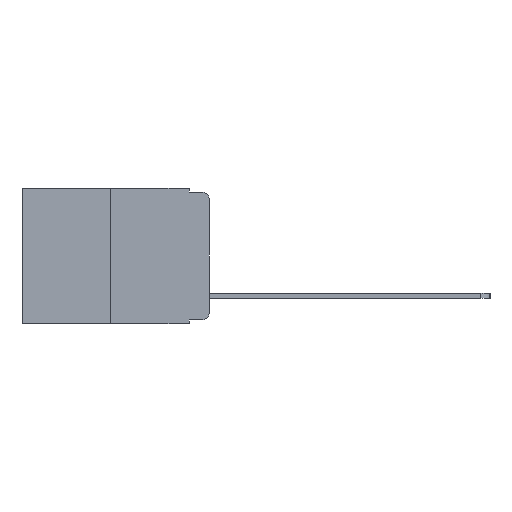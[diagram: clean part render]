
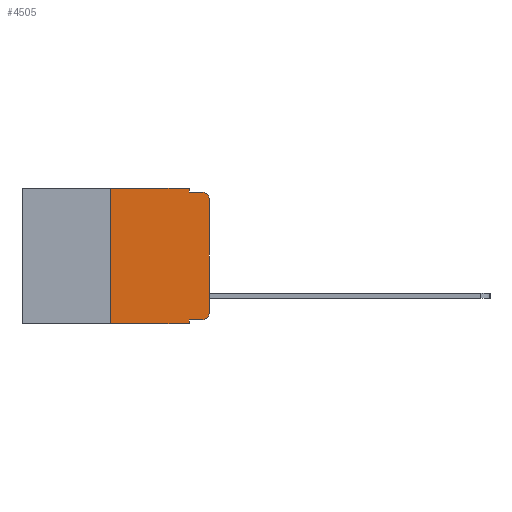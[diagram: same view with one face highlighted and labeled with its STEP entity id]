
A CAD part, left-side view. The second image highlights one B-rep face of the part: STEP entity #4505.
In plain terms, the highlighted planar face has unit normal (-1, 0, 0).
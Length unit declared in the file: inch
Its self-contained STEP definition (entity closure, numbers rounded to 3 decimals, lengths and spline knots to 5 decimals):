
#16 = EDGE_CURVE ( 'NONE', #2406, #8266, #8971, .T. ) ;
#35 = VERTEX_POINT ( 'NONE', #897 ) ;
#114 = ORIENTED_EDGE ( 'NONE', *, *, #5518, .F. ) ;
#208 = AXIS2_PLACEMENT_3D ( 'NONE', #2878, #8961, #3719 ) ;
#295 = CARTESIAN_POINT ( 'NONE',  ( 0., 0.051, 0. ) ) ;
#467 = ORIENTED_EDGE ( 'NONE', *, *, #7048, .F. ) ;
#675 = EDGE_CURVE ( 'NONE', #3174, #8266, #1093, .T. ) ;
#722 = VECTOR ( 'NONE', #9252, 39.37008 ) ;
#881 = LINE ( 'NONE', #295, #9978 ) ;
#897 = CARTESIAN_POINT ( 'NONE',  ( 0., 0.25, 0. ) ) ;
#975 = EDGE_CURVE ( 'NONE', #2092, #35, #4726, .T. ) ;
#1050 = LINE ( 'NONE', #3229, #722 ) ;
#1093 = LINE ( 'NONE', #2031, #4134 ) ;
#1581 = CARTESIAN_POINT ( 'NONE',  ( 0., 0.051, -0.333 ) ) ;
#2031 = CARTESIAN_POINT ( 'NONE',  ( 0., 0.051, -0.01 ) ) ;
#2092 = VERTEX_POINT ( 'NONE', #10854 ) ;
#2406 = VERTEX_POINT ( 'NONE', #10140 ) ;
#2514 = DIRECTION ( 'NONE',  ( 0., -1., 0. ) ) ;
#2523 = VERTEX_POINT ( 'NONE', #6070 ) ;
#2529 = CARTESIAN_POINT ( 'NONE',  ( 0., 0.051, -0.01 ) ) ;
#2704 = VECTOR ( 'NONE', #10367, 39.37008 ) ;
#2850 = ORIENTED_EDGE ( 'NONE', *, *, #3019, .F. ) ;
#2878 = CARTESIAN_POINT ( 'NONE',  ( 0., 0.02, -0.03 ) ) ;
#2907 = LINE ( 'NONE', #9374, #11278 ) ;
#2908 = DIRECTION ( 'NONE',  ( 0., -1., 0. ) ) ;
#3019 = EDGE_CURVE ( 'NONE', #9167, #3174, #881, .T. ) ;
#3174 = VERTEX_POINT ( 'NONE', #2529 ) ;
#3229 = CARTESIAN_POINT ( 'NONE',  ( 0., 0., 0. ) ) ;
#3245 = AXIS2_PLACEMENT_3D ( 'NONE', #5393, #3585, #8828 ) ;
#3280 = DIRECTION ( 'NONE',  ( -1., 0., 0. ) ) ;
#3315 = CARTESIAN_POINT ( 'NONE',  ( 0., 0.02, -0.313 ) ) ;
#3332 = VERTEX_POINT ( 'NONE', #1581 ) ;
#3585 = DIRECTION ( 'NONE',  ( 1., 0., 0. ) ) ;
#3594 = AXIS2_PLACEMENT_3D ( 'NONE', #3315, #3280, #9082 ) ;
#3719 = DIRECTION ( 'NONE',  ( 0., 0., -1. ) ) ;
#3962 = EDGE_CURVE ( 'NONE', #3332, #2523, #2907, .T. ) ;
#4134 = VECTOR ( 'NONE', #10295, 39.37008 ) ;
#4366 = FACE_OUTER_BOUND ( 'NONE', #8777, .T. ) ;
#4473 = CARTESIAN_POINT ( 'NONE',  ( 0., 0.051, 0. ) ) ;
#4491 = VECTOR ( 'NONE', #2514, 39.37008 ) ;
#4505 = ADVANCED_FACE ( 'NONE', ( #4366 ), #11149, .F. ) ;
#4626 = DIRECTION ( 'NONE',  ( 0., 0., 1. ) ) ;
#4726 = LINE ( 'NONE', #6317, #6840 ) ;
#4742 = LINE ( 'NONE', #9960, #11116 ) ;
#4773 = LINE ( 'NONE', #8956, #4491 ) ;
#4968 = EDGE_CURVE ( 'NONE', #2523, #9994, #10797, .T. ) ;
#5227 = CARTESIAN_POINT ( 'NONE',  ( 0., 0.02, -0.01 ) ) ;
#5393 = CARTESIAN_POINT ( 'NONE',  ( 0., 0.473, 0. ) ) ;
#5518 = EDGE_CURVE ( 'NONE', #35, #9167, #4773, .T. ) ;
#6070 = CARTESIAN_POINT ( 'NONE',  ( 0., 0.02, -0.333 ) ) ;
#6317 = CARTESIAN_POINT ( 'NONE',  ( 0., 0.25, 0. ) ) ;
#6396 = CARTESIAN_POINT ( 'NONE',  ( 0., 0.051, 0. ) ) ;
#6840 = VECTOR ( 'NONE', #4626, 39.37008 ) ;
#7048 = EDGE_CURVE ( 'NONE', #3332, #8185, #9332, .T. ) ;
#7272 = ORIENTED_EDGE ( 'NONE', *, *, #675, .F. ) ;
#7359 = DIRECTION ( 'NONE',  ( 0., -1., 0. ) ) ;
#7493 = EDGE_CURVE ( 'NONE', #2092, #8185, #4742, .T. ) ;
#7540 = ORIENTED_EDGE ( 'NONE', *, *, #7493, .T. ) ;
#8185 = VERTEX_POINT ( 'NONE', #9365 ) ;
#8266 = VERTEX_POINT ( 'NONE', #5227 ) ;
#8311 = ORIENTED_EDGE ( 'NONE', *, *, #3962, .T. ) ;
#8777 = EDGE_LOOP ( 'NONE', ( #11228, #9442, #7272, #2850, #114, #9687, #7540, #467, #8311, #10399 ) ) ;
#8828 = DIRECTION ( 'NONE',  ( 0., 0., -1. ) ) ;
#8846 = CARTESIAN_POINT ( 'NONE',  ( 0., 0., -0.313 ) ) ;
#8956 = CARTESIAN_POINT ( 'NONE',  ( 0., 0.473, 0. ) ) ;
#8961 = DIRECTION ( 'NONE',  ( -1., 0., 0. ) ) ;
#8971 = CIRCLE ( 'NONE', #208, 0.02 ) ;
#9082 = DIRECTION ( 'NONE',  ( 0., 0., -1. ) ) ;
#9167 = VERTEX_POINT ( 'NONE', #6396 ) ;
#9252 = DIRECTION ( 'NONE',  ( 0., 0., 1. ) ) ;
#9332 = LINE ( 'NONE', #4473, #2704 ) ;
#9365 = CARTESIAN_POINT ( 'NONE',  ( 0., 0.051, -0.343 ) ) ;
#9374 = CARTESIAN_POINT ( 'NONE',  ( 0., 0.051, -0.333 ) ) ;
#9442 = ORIENTED_EDGE ( 'NONE', *, *, #16, .T. ) ;
#9687 = ORIENTED_EDGE ( 'NONE', *, *, #975, .F. ) ;
#9960 = CARTESIAN_POINT ( 'NONE',  ( 0., 0.473, -0.343 ) ) ;
#9978 = VECTOR ( 'NONE', #10283, 39.37008 ) ;
#9994 = VERTEX_POINT ( 'NONE', #8846 ) ;
#10140 = CARTESIAN_POINT ( 'NONE',  ( 0., 0., -0.03 ) ) ;
#10283 = DIRECTION ( 'NONE',  ( 0., 0., -1. ) ) ;
#10295 = DIRECTION ( 'NONE',  ( 0., -1., 0. ) ) ;
#10367 = DIRECTION ( 'NONE',  ( 0., 0., -1. ) ) ;
#10399 = ORIENTED_EDGE ( 'NONE', *, *, #4968, .T. ) ;
#10497 = EDGE_CURVE ( 'NONE', #9994, #2406, #1050, .T. ) ;
#10797 = CIRCLE ( 'NONE', #3594, 0.02 ) ;
#10854 = CARTESIAN_POINT ( 'NONE',  ( 0., 0.25, -0.343 ) ) ;
#11116 = VECTOR ( 'NONE', #7359, 39.37008 ) ;
#11149 = PLANE ( 'NONE',  #3245 ) ;
#11228 = ORIENTED_EDGE ( 'NONE', *, *, #10497, .T. ) ;
#11278 = VECTOR ( 'NONE', #2908, 39.37008 ) ;
